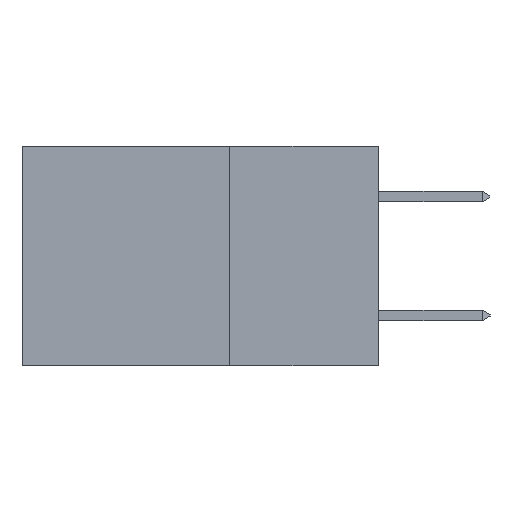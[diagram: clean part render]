
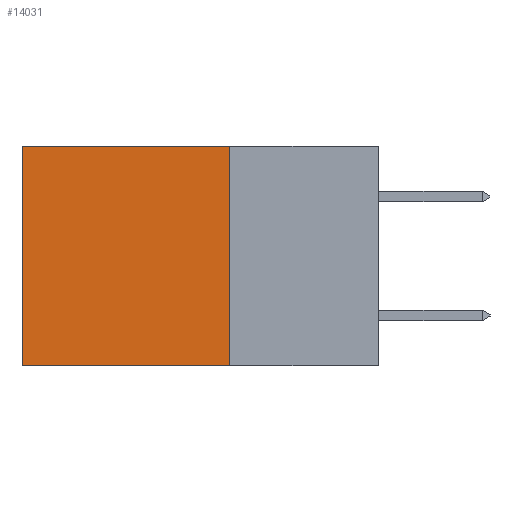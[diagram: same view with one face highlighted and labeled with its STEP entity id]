
A CAD part, left-side view. The second image highlights one B-rep face of the part: STEP entity #14031.
In plain terms, the highlighted planar face has unit normal (-1, 0, 0).
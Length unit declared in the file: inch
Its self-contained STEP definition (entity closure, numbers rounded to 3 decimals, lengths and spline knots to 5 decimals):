
#42 = CARTESIAN_POINT ( 'NONE',  ( 0.2615, 0.25, -0.37 ) ) ;
#49 = VERTEX_POINT ( 'NONE', #888 ) ;
#78 = EDGE_CURVE ( 'NONE', #5655, #6443, #8812, .T. ) ;
#440 = VECTOR ( 'NONE', #8166, 39.37008 ) ;
#882 = ORIENTED_EDGE ( 'NONE', *, *, #12893, .F. ) ;
#888 = CARTESIAN_POINT ( 'NONE',  ( 0.2615, 0.25, 0. ) ) ;
#2856 = DIRECTION ( 'NONE',  ( 0., 0., -1. ) ) ;
#2990 = LINE ( 'NONE', #7756, #3417 ) ;
#3046 = EDGE_CURVE ( 'NONE', #49, #5655, #2990, .T. ) ;
#3417 = VECTOR ( 'NONE', #8159, 39.37008 ) ;
#3940 = VECTOR ( 'NONE', #4390, 39.37008 ) ;
#4318 = ORIENTED_EDGE ( 'NONE', *, *, #15313, .F. ) ;
#4390 = DIRECTION ( 'NONE',  ( 0., 0., -1. ) ) ;
#4715 = CARTESIAN_POINT ( 'NONE',  ( 0.2615, 0.6, 0. ) ) ;
#4765 = CARTESIAN_POINT ( 'NONE',  ( 0.2615, 0.6, -0.37 ) ) ;
#5220 = ORIENTED_EDGE ( 'NONE', *, *, #3046, .T. ) ;
#5655 = VERTEX_POINT ( 'NONE', #4715 ) ;
#6443 = VERTEX_POINT ( 'NONE', #4765 ) ;
#7642 = CARTESIAN_POINT ( 'NONE',  ( 0.2615, 0.25, -0.37 ) ) ;
#7756 = CARTESIAN_POINT ( 'NONE',  ( 0.2615, 0.25, 0. ) ) ;
#8159 = DIRECTION ( 'NONE',  ( 0., 1., 0. ) ) ;
#8166 = DIRECTION ( 'NONE',  ( 0., 0., -1. ) ) ;
#8362 = LINE ( 'NONE', #7642, #12022 ) ;
#8609 = CARTESIAN_POINT ( 'NONE',  ( 0.2615, 0.25, -0.37 ) ) ;
#8812 = LINE ( 'NONE', #11268, #440 ) ;
#9066 = DIRECTION ( 'NONE',  ( 0., 1., 0. ) ) ;
#9880 = PLANE ( 'NONE',  #15225 ) ;
#10995 = LINE ( 'NONE', #8609, #3940 ) ;
#11063 = CARTESIAN_POINT ( 'NONE',  ( 0.2615, 0.25, -0.37 ) ) ;
#11086 = ORIENTED_EDGE ( 'NONE', *, *, #78, .T. ) ;
#11268 = CARTESIAN_POINT ( 'NONE',  ( 0.2615, 0.6, -0.37 ) ) ;
#11272 = DIRECTION ( 'NONE',  ( 1., 0., 0. ) ) ;
#11355 = VERTEX_POINT ( 'NONE', #11063 ) ;
#12022 = VECTOR ( 'NONE', #9066, 39.37008 ) ;
#12893 = EDGE_CURVE ( 'NONE', #11355, #6443, #8362, .T. ) ;
#13312 = FACE_OUTER_BOUND ( 'NONE', #14392, .T. ) ;
#14031 = ADVANCED_FACE ( 'NONE', ( #13312 ), #9880, .F. ) ;
#14392 = EDGE_LOOP ( 'NONE', ( #11086, #882, #4318, #5220 ) ) ;
#15225 = AXIS2_PLACEMENT_3D ( 'NONE', #42, #11272, #2856 ) ;
#15313 = EDGE_CURVE ( 'NONE', #49, #11355, #10995, .T. ) ;
